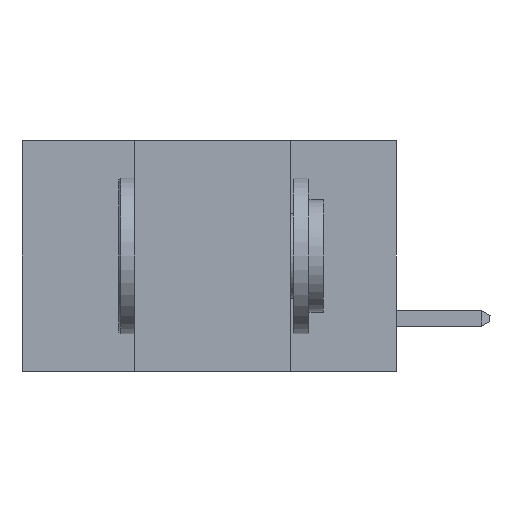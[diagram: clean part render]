
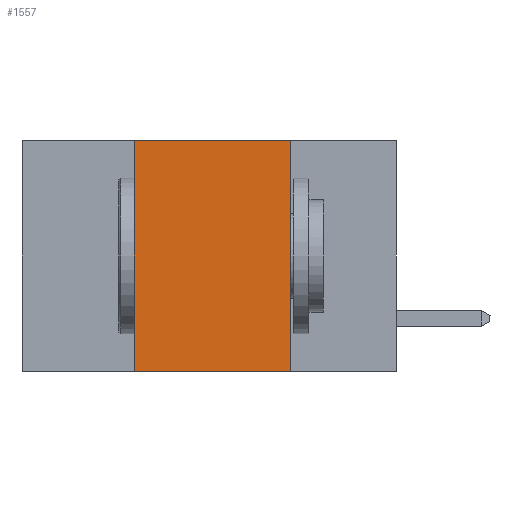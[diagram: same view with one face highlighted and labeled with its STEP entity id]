
A CAD part, left-side view. The second image highlights one B-rep face of the part: STEP entity #1557.
In plain terms, the highlighted planar face has unit normal (-1, 0, 0).
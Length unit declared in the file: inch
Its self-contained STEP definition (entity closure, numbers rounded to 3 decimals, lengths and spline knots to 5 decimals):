
#165 = DIRECTION ( 'NONE',  ( 0., -1., 0. ) ) ;
#428 = LINE ( 'NONE', #4162, #9842 ) ;
#772 = LINE ( 'NONE', #1449, #3547 ) ;
#1040 = DIRECTION ( 'NONE',  ( 0., 0., -1. ) ) ;
#1209 = EDGE_LOOP ( 'NONE', ( #1377, #1576, #9127, #3191 ) ) ;
#1377 = ORIENTED_EDGE ( 'NONE', *, *, #4469, .F. ) ;
#1449 = CARTESIAN_POINT ( 'NONE',  ( 0., 0.42, 0. ) ) ;
#1557 = ADVANCED_FACE ( 'NONE', ( #7783 ), #9421, .F. ) ;
#1576 = ORIENTED_EDGE ( 'NONE', *, *, #2528, .F. ) ;
#1885 = CARTESIAN_POINT ( 'NONE',  ( 0., 0.42, 0. ) ) ;
#2301 = LINE ( 'NONE', #6667, #8784 ) ;
#2528 = EDGE_CURVE ( 'NONE', #7774, #9646, #428, .T. ) ;
#2760 = EDGE_CURVE ( 'NONE', #5596, #7774, #772, .T. ) ;
#3191 = ORIENTED_EDGE ( 'NONE', *, *, #9177, .T. ) ;
#3547 = VECTOR ( 'NONE', #6365, 39.37008 ) ;
#3668 = VECTOR ( 'NONE', #5614, 39.37008 ) ;
#4162 = CARTESIAN_POINT ( 'NONE',  ( 0., 0.6, 0. ) ) ;
#4397 = VERTEX_POINT ( 'NONE', #4910 ) ;
#4469 = EDGE_CURVE ( 'NONE', #9646, #4397, #2301, .T. ) ;
#4910 = CARTESIAN_POINT ( 'NONE',  ( 0., 0.17, -0.37 ) ) ;
#5313 = CARTESIAN_POINT ( 'NONE',  ( 0., 0.6, 0. ) ) ;
#5596 = VERTEX_POINT ( 'NONE', #5916 ) ;
#5614 = DIRECTION ( 'NONE',  ( 0., -1., 0. ) ) ;
#5671 = DIRECTION ( 'NONE',  ( 0., 0., -1. ) ) ;
#5916 = CARTESIAN_POINT ( 'NONE',  ( 0., 0.42, -0.37 ) ) ;
#6365 = DIRECTION ( 'NONE',  ( 0., 0., 1. ) ) ;
#6390 = DIRECTION ( 'NONE',  ( 1., 0., 0. ) ) ;
#6634 = LINE ( 'NONE', #8833, #3668 ) ;
#6667 = CARTESIAN_POINT ( 'NONE',  ( 0., 0.17, 0. ) ) ;
#7645 = AXIS2_PLACEMENT_3D ( 'NONE', #5313, #6390, #5671 ) ;
#7774 = VERTEX_POINT ( 'NONE', #1885 ) ;
#7783 = FACE_OUTER_BOUND ( 'NONE', #1209, .T. ) ;
#8784 = VECTOR ( 'NONE', #1040, 39.37008 ) ;
#8833 = CARTESIAN_POINT ( 'NONE',  ( 0., 0.6, -0.37 ) ) ;
#9127 = ORIENTED_EDGE ( 'NONE', *, *, #2760, .F. ) ;
#9177 = EDGE_CURVE ( 'NONE', #5596, #4397, #6634, .T. ) ;
#9421 = PLANE ( 'NONE',  #7645 ) ;
#9646 = VERTEX_POINT ( 'NONE', #9804 ) ;
#9804 = CARTESIAN_POINT ( 'NONE',  ( 0., 0.17, 0. ) ) ;
#9842 = VECTOR ( 'NONE', #165, 39.37008 ) ;
